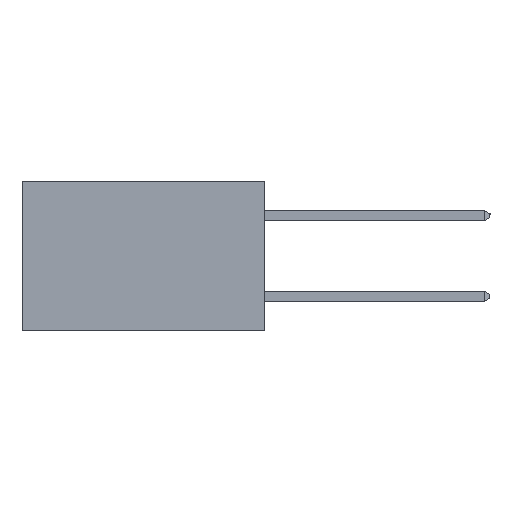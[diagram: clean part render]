
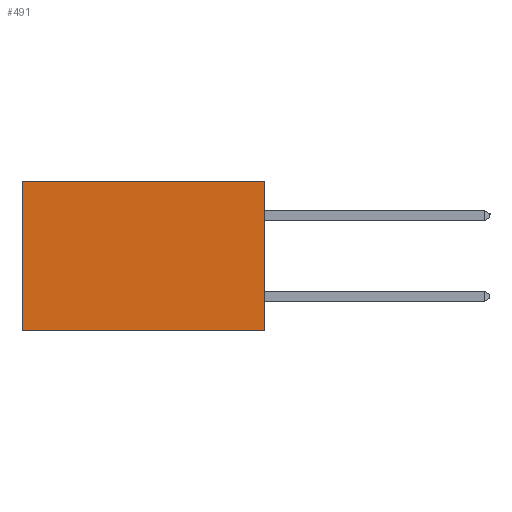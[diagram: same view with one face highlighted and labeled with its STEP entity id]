
A CAD part, left-side view. The second image highlights one B-rep face of the part: STEP entity #491.
In plain terms, the highlighted planar face has unit normal (-1, 0, 0).
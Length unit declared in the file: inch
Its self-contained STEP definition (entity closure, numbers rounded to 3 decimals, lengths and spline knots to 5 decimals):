
#491 = ADVANCED_FACE ( 'NONE', ( #17832 ), #19728, .F. ) ;
#1665 = DIRECTION ( 'NONE',  ( 0., 0., -1. ) ) ;
#1863 = DIRECTION ( 'NONE',  ( 0., 1., 0. ) ) ;
#2172 = LINE ( 'NONE', #20364, #7659 ) ;
#3171 = DIRECTION ( 'NONE',  ( 0., 0., -1. ) ) ;
#3288 = CARTESIAN_POINT ( 'NONE',  ( 0.2615, 0., -0.37 ) ) ;
#3556 = DIRECTION ( 'NONE',  ( 1., 0., 0. ) ) ;
#3975 = VERTEX_POINT ( 'NONE', #10728 ) ;
#7659 = VECTOR ( 'NONE', #7855, 39.37008 ) ;
#7813 = AXIS2_PLACEMENT_3D ( 'NONE', #3288, #3556, #1665 ) ;
#7855 = DIRECTION ( 'NONE',  ( 0., 1., 0. ) ) ;
#8578 = ORIENTED_EDGE ( 'NONE', *, *, #24777, .T. ) ;
#8965 = ORIENTED_EDGE ( 'NONE', *, *, #11617, .F. ) ;
#9430 = ORIENTED_EDGE ( 'NONE', *, *, #20239, .F. ) ;
#10728 = CARTESIAN_POINT ( 'NONE',  ( 0.2615, 0.6, -0.37 ) ) ;
#10910 = VERTEX_POINT ( 'NONE', #21123 ) ;
#11617 = EDGE_CURVE ( 'NONE', #10910, #3975, #2172, .T. ) ;
#12094 = EDGE_CURVE ( 'NONE', #20741, #23450, #22229, .T. ) ;
#13930 = CARTESIAN_POINT ( 'NONE',  ( 0.2615, 0., -0.37 ) ) ;
#14012 = VECTOR ( 'NONE', #3171, 39.37008 ) ;
#14540 = ORIENTED_EDGE ( 'NONE', *, *, #12094, .T. ) ;
#14825 = DIRECTION ( 'NONE',  ( 0., 0., -1. ) ) ;
#15214 = LINE ( 'NONE', #23471, #23169 ) ;
#17677 = CARTESIAN_POINT ( 'NONE',  ( 0.2615, 0., 0. ) ) ;
#17832 = FACE_OUTER_BOUND ( 'NONE', #21001, .T. ) ;
#18700 = CARTESIAN_POINT ( 'NONE',  ( 0.2615, 0., 0. ) ) ;
#19728 = PLANE ( 'NONE',  #7813 ) ;
#20239 = EDGE_CURVE ( 'NONE', #20741, #10910, #22058, .T. ) ;
#20364 = CARTESIAN_POINT ( 'NONE',  ( 0.2615, 0., -0.37 ) ) ;
#20741 = VERTEX_POINT ( 'NONE', #17677 ) ;
#21001 = EDGE_LOOP ( 'NONE', ( #8578, #8965, #9430, #14540 ) ) ;
#21123 = CARTESIAN_POINT ( 'NONE',  ( 0.2615, 0., -0.37 ) ) ;
#22058 = LINE ( 'NONE', #13930, #14012 ) ;
#22229 = LINE ( 'NONE', #18700, #25039 ) ;
#23169 = VECTOR ( 'NONE', #14825, 39.37008 ) ;
#23450 = VERTEX_POINT ( 'NONE', #24277 ) ;
#23471 = CARTESIAN_POINT ( 'NONE',  ( 0.2615, 0.6, -0.37 ) ) ;
#24277 = CARTESIAN_POINT ( 'NONE',  ( 0.2615, 0.6, 0. ) ) ;
#24777 = EDGE_CURVE ( 'NONE', #23450, #3975, #15214, .T. ) ;
#25039 = VECTOR ( 'NONE', #1863, 39.37008 ) ;
